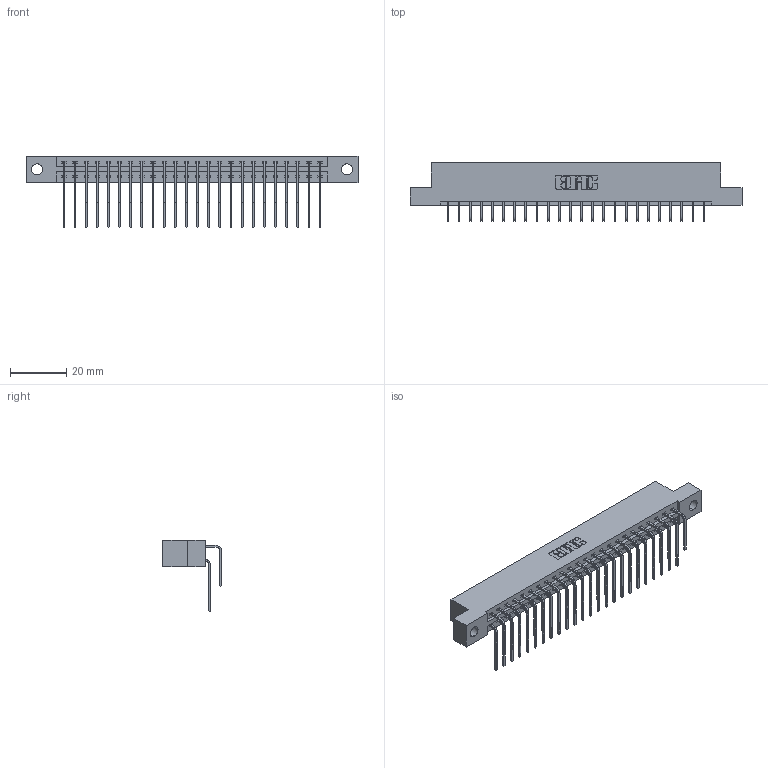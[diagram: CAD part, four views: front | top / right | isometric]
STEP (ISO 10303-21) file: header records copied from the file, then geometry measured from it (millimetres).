
FILE_DESCRIPTION (( 'STEP AP203' ), '1' );
FILE_NAME ('387-048-559-204.STEP', '2019-10-18T10:52:33', ( '' ), ( '' ), 'SwSTEP 2.0', 'SolidWorks 2016', '' );
FILE_SCHEMA (( 'CONFIG_CONTROL_DESIGN' ));
Length unit declared in the file: inch
Products named in the file (4): 387-048-559-204; 345-292-001_558 559 Tail - 1; 345-292-001_559 Tail - 2; 337 Part_Flush Mounting Lugs - 0.156 Dia-TH
Assembly tree (49 placements, depth 2):
  387-048-559-204
    337 Part_Flush Mounting Lugs - 0.156 Dia-TH
    345-292-001_558 559 Tail - 1  x24
    345-292-001_559 Tail - 2  x24
Bounding box: 118.11 x 20.9 x 25.53 mm (x, y, z)
Volume: 12396.8 mm3; surface area: 15027.5 mm2
Topology: 49 solids, 49 shells, 2802 faces, 8327 edges, 5486 vertices
Faces by surface type: plane 1990, cylinder 812
Entity records: 22723 total; most frequent: CARTESIAN_POINT 3889, ORIENTED_EDGE 3774, DIRECTION 3323, EDGE_CURVE 1887, LINE 1719, VECTOR 1719, VERTEX_POINT 1254, AXIS2_PLACEMENT_3D 802
